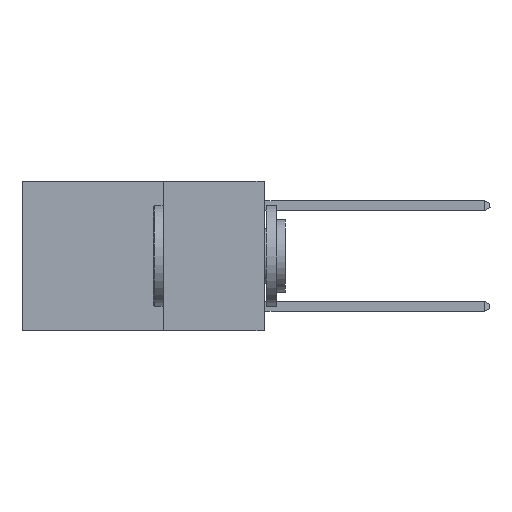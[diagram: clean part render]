
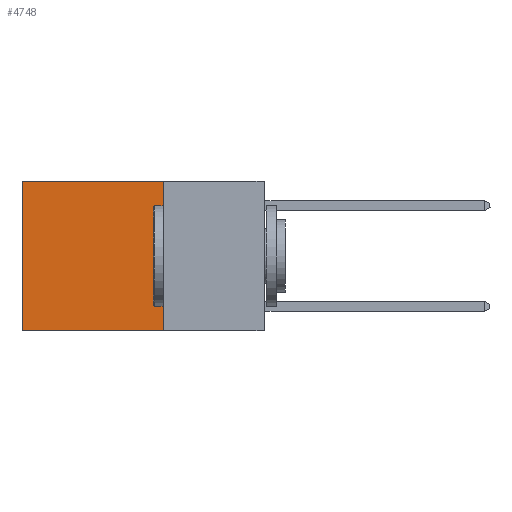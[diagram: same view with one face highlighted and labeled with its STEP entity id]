
A CAD part, left-side view. The second image highlights one B-rep face of the part: STEP entity #4748.
In plain terms, the highlighted planar face has unit normal (-1, 0, 0).
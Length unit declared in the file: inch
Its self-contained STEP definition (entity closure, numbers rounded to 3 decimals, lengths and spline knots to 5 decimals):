
#79 = CARTESIAN_POINT ( 'NONE',  ( 0.2625, 0.6, -0.37 ) ) ;
#344 = DIRECTION ( 'NONE',  ( 0., 1., 0. ) ) ;
#944 = VERTEX_POINT ( 'NONE', #79 ) ;
#1688 = FACE_OUTER_BOUND ( 'NONE', #9233, .T. ) ;
#2491 = LINE ( 'NONE', #8762, #7650 ) ;
#3822 = VERTEX_POINT ( 'NONE', #10745 ) ;
#4002 = DIRECTION ( 'NONE',  ( 1., 0., 0. ) ) ;
#4643 = ORIENTED_EDGE ( 'NONE', *, *, #7267, .F. ) ;
#4748 = ADVANCED_FACE ( 'NONE', ( #1688 ), #12423, .F. ) ;
#4973 = DIRECTION ( 'NONE',  ( 0., 0., -1. ) ) ;
#5153 = LINE ( 'NONE', #5229, #12901 ) ;
#5229 = CARTESIAN_POINT ( 'NONE',  ( 0.2625, 0.6, 0. ) ) ;
#6660 = CARTESIAN_POINT ( 'NONE',  ( 0.2625, 0.25, 0. ) ) ;
#7267 = EDGE_CURVE ( 'NONE', #12696, #944, #2491, .T. ) ;
#7650 = VECTOR ( 'NONE', #344, 39.37008 ) ;
#7977 = ORIENTED_EDGE ( 'NONE', *, *, #13885, .T. ) ;
#8621 = DIRECTION ( 'NONE',  ( 0., 0., -1. ) ) ;
#8762 = CARTESIAN_POINT ( 'NONE',  ( 0.2625, 0.25, -0.37 ) ) ;
#9220 = CARTESIAN_POINT ( 'NONE',  ( 0.2625, 0.25, 0. ) ) ;
#9233 = EDGE_LOOP ( 'NONE', ( #7977, #4643, #9644, #13585 ) ) ;
#9520 = EDGE_CURVE ( 'NONE', #11724, #3822, #12557, .T. ) ;
#9644 = ORIENTED_EDGE ( 'NONE', *, *, #11640, .F. ) ;
#10338 = CARTESIAN_POINT ( 'NONE',  ( 0.2625, 0.25, -0.37 ) ) ;
#10745 = CARTESIAN_POINT ( 'NONE',  ( 0.2625, 0.6, 0. ) ) ;
#11002 = VECTOR ( 'NONE', #13538, 39.37008 ) ;
#11484 = CARTESIAN_POINT ( 'NONE',  ( 0.2625, 0.25, 0. ) ) ;
#11640 = EDGE_CURVE ( 'NONE', #11724, #12696, #13129, .T. ) ;
#11724 = VERTEX_POINT ( 'NONE', #13900 ) ;
#12160 = DIRECTION ( 'NONE',  ( 0., 0., -1. ) ) ;
#12406 = AXIS2_PLACEMENT_3D ( 'NONE', #11484, #4002, #4973 ) ;
#12423 = PLANE ( 'NONE',  #12406 ) ;
#12557 = LINE ( 'NONE', #9220, #11002 ) ;
#12696 = VERTEX_POINT ( 'NONE', #10338 ) ;
#12901 = VECTOR ( 'NONE', #8621, 39.37008 ) ;
#13129 = LINE ( 'NONE', #6660, #13293 ) ;
#13293 = VECTOR ( 'NONE', #12160, 39.37008 ) ;
#13538 = DIRECTION ( 'NONE',  ( 0., 1., 0. ) ) ;
#13585 = ORIENTED_EDGE ( 'NONE', *, *, #9520, .T. ) ;
#13885 = EDGE_CURVE ( 'NONE', #3822, #944, #5153, .T. ) ;
#13900 = CARTESIAN_POINT ( 'NONE',  ( 0.2625, 0.25, 0. ) ) ;
